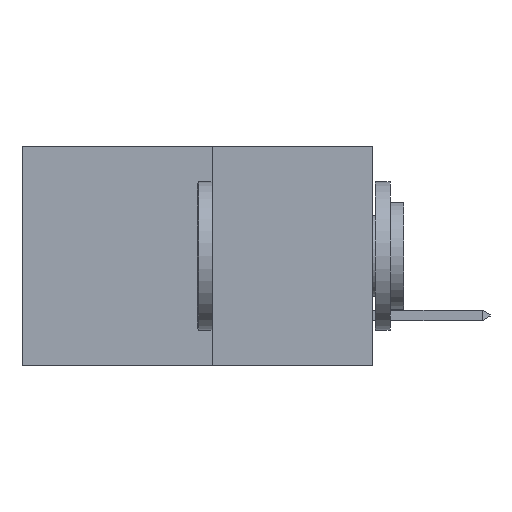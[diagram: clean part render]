
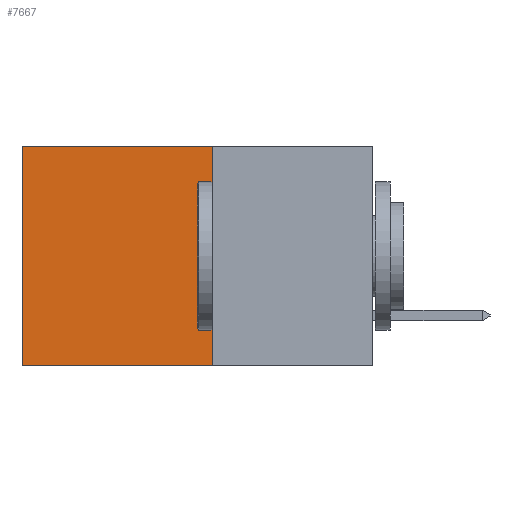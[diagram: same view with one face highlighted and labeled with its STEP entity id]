
A CAD part, left-side view. The second image highlights one B-rep face of the part: STEP entity #7667.
In plain terms, the highlighted planar face has unit normal (-1, 0, 0).
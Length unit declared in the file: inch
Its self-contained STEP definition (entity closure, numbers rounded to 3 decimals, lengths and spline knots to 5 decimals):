
#390 = VERTEX_POINT ( 'NONE', #4249 ) ;
#1524 = VERTEX_POINT ( 'NONE', #4274 ) ;
#2127 = EDGE_CURVE ( 'NONE', #390, #4657, #5947, .T. ) ;
#2133 = DIRECTION ( 'NONE',  ( 0., 0., -1. ) ) ;
#2327 = VECTOR ( 'NONE', #2133, 39.37008 ) ;
#2626 = ORIENTED_EDGE ( 'NONE', *, *, #15144, .T. ) ;
#2779 = ORIENTED_EDGE ( 'NONE', *, *, #10864, .F. ) ;
#3022 = EDGE_CURVE ( 'NONE', #1524, #15623, #15923, .T. ) ;
#4114 = CARTESIAN_POINT ( 'NONE',  ( 0.277, 0.27, 0. ) ) ;
#4249 = CARTESIAN_POINT ( 'NONE',  ( 0.277, 0.59, 0. ) ) ;
#4274 = CARTESIAN_POINT ( 'NONE',  ( 0.277, 0.27, 0. ) ) ;
#4657 = VERTEX_POINT ( 'NONE', #17051 ) ;
#5839 = LINE ( 'NONE', #4114, #16271 ) ;
#5947 = LINE ( 'NONE', #15400, #2327 ) ;
#6046 = ORIENTED_EDGE ( 'NONE', *, *, #2127, .T. ) ;
#6940 = LINE ( 'NONE', #9154, #9699 ) ;
#7055 = CARTESIAN_POINT ( 'NONE',  ( 0.277, 0.27, -0.37 ) ) ;
#7667 = ADVANCED_FACE ( 'NONE', ( #10655 ), #12807, .F. ) ;
#8679 = VECTOR ( 'NONE', #16426, 39.37008 ) ;
#8716 = DIRECTION ( 'NONE',  ( 0., 0., -1. ) ) ;
#9038 = AXIS2_PLACEMENT_3D ( 'NONE', #15506, #16872, #8716 ) ;
#9154 = CARTESIAN_POINT ( 'NONE',  ( 0.277, 0.27, -0.37 ) ) ;
#9699 = VECTOR ( 'NONE', #10531, 39.37008 ) ;
#10531 = DIRECTION ( 'NONE',  ( 0., 1., 0. ) ) ;
#10655 = FACE_OUTER_BOUND ( 'NONE', #16730, .T. ) ;
#10864 = EDGE_CURVE ( 'NONE', #15623, #4657, #6940, .T. ) ;
#10870 = ORIENTED_EDGE ( 'NONE', *, *, #3022, .F. ) ;
#12297 = DIRECTION ( 'NONE',  ( 0., 1., 0. ) ) ;
#12807 = PLANE ( 'NONE',  #9038 ) ;
#15144 = EDGE_CURVE ( 'NONE', #1524, #390, #5839, .T. ) ;
#15400 = CARTESIAN_POINT ( 'NONE',  ( 0.277, 0.59, -0.37 ) ) ;
#15506 = CARTESIAN_POINT ( 'NONE',  ( 0.277, 0.27, -0.37 ) ) ;
#15623 = VERTEX_POINT ( 'NONE', #7055 ) ;
#15923 = LINE ( 'NONE', #16773, #8679 ) ;
#16271 = VECTOR ( 'NONE', #12297, 39.37008 ) ;
#16426 = DIRECTION ( 'NONE',  ( 0., 0., -1. ) ) ;
#16730 = EDGE_LOOP ( 'NONE', ( #6046, #2779, #10870, #2626 ) ) ;
#16773 = CARTESIAN_POINT ( 'NONE',  ( 0.277, 0.27, -0.37 ) ) ;
#16872 = DIRECTION ( 'NONE',  ( 1., 0., 0. ) ) ;
#17051 = CARTESIAN_POINT ( 'NONE',  ( 0.277, 0.59, -0.37 ) ) ;
